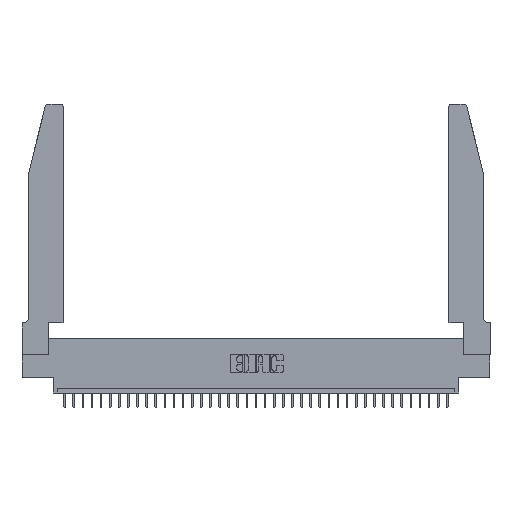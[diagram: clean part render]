
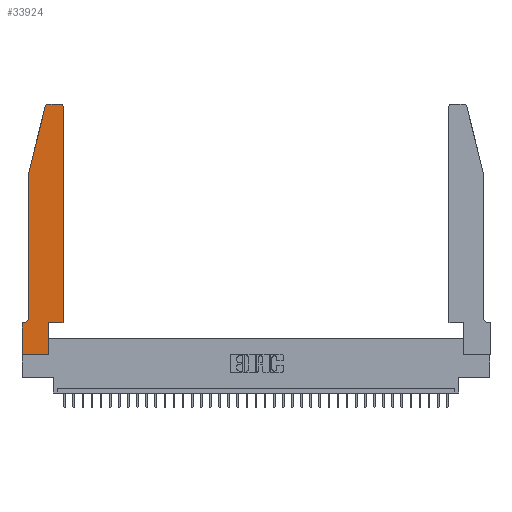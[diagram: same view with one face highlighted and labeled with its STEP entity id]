
A CAD part, top view. The second image highlights one B-rep face of the part: STEP entity #33924.
In plain terms, the highlighted planar face has unit normal (0, 0, 1).
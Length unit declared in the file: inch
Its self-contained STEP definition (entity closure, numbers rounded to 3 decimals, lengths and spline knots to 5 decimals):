
#846 = VECTOR ( 'NONE', #14399, 39.37008 ) ;
#1348 = LINE ( 'NONE', #17926, #846 ) ;
#2010 = EDGE_CURVE ( 'NONE', #20966, #9836, #18741, .T. ) ;
#2054 = CARTESIAN_POINT ( 'NONE',  ( 0.4205, 2.75, 0.37 ) ) ;
#2552 = LINE ( 'NONE', #18133, #14204 ) ;
#2618 = CARTESIAN_POINT ( 'NONE',  ( 0.0055, 0.35, 0.37 ) ) ;
#2732 = AXIS2_PLACEMENT_3D ( 'NONE', #2826, #20329, #20874 ) ;
#2826 = CARTESIAN_POINT ( 'NONE',  ( 0.4205, 2.72, 0.37 ) ) ;
#3093 = VECTOR ( 'NONE', #26132, 39.37008 ) ;
#3530 = CARTESIAN_POINT ( 'NONE',  ( 0.284, 2.75, 0.37 ) ) ;
#3638 = ORIENTED_EDGE ( 'NONE', *, *, #16015, .T. ) ;
#3653 = EDGE_CURVE ( 'NONE', #21396, #20966, #22659, .T. ) ;
#4939 = CARTESIAN_POINT ( 'NONE',  ( 0.2865, 0.35, 0.37 ) ) ;
#5002 = CIRCLE ( 'NONE', #24371, 0.03 ) ;
#5201 = ORIENTED_EDGE ( 'NONE', *, *, #29090, .T. ) ;
#6491 = LINE ( 'NONE', #16230, #36159 ) ;
#6563 = DIRECTION ( 'NONE',  ( 1., 0., 0. ) ) ;
#7030 = ORIENTED_EDGE ( 'NONE', *, *, #3653, .T. ) ;
#7491 = CARTESIAN_POINT ( 'NONE',  ( 0.25487, 2.72718, 0.37 ) ) ;
#7581 = EDGE_CURVE ( 'NONE', #14139, #18586, #10402, .T. ) ;
#7671 = VERTEX_POINT ( 'NONE', #10787 ) ;
#7734 = DIRECTION ( 'NONE',  ( 0., 1., 0. ) ) ;
#7738 = VECTOR ( 'NONE', #16692, 39.37008 ) ;
#8858 = ORIENTED_EDGE ( 'NONE', *, *, #12241, .T. ) ;
#9411 = EDGE_CURVE ( 'NONE', #30691, #10768, #2552, .T. ) ;
#9836 = VERTEX_POINT ( 'NONE', #35978 ) ;
#10402 = LINE ( 'NONE', #25443, #3093 ) ;
#10768 = VERTEX_POINT ( 'NONE', #25548 ) ;
#10787 = CARTESIAN_POINT ( 'NONE',  ( 0.0755, 2., 0.37 ) ) ;
#10963 = DIRECTION ( 'NONE',  ( 0., -1., 0. ) ) ;
#12241 = EDGE_CURVE ( 'NONE', #14148, #30691, #15282, .T. ) ;
#13136 = LINE ( 'NONE', #33552, #36939 ) ;
#13427 = EDGE_CURVE ( 'NONE', #31234, #14148, #1348, .T. ) ;
#14139 = VERTEX_POINT ( 'NONE', #2054 ) ;
#14148 = VERTEX_POINT ( 'NONE', #20504 ) ;
#14204 = VECTOR ( 'NONE', #6563, 39.37008 ) ;
#14399 = DIRECTION ( 'NONE',  ( 1., 0., 0. ) ) ;
#14471 = EDGE_CURVE ( 'NONE', #7671, #21396, #21504, .T. ) ;
#14508 = VERTEX_POINT ( 'NONE', #20963 ) ;
#14814 = CARTESIAN_POINT ( 'NONE',  ( 0.0055, 0.42, 0.37 ) ) ;
#14862 = DIRECTION ( 'NONE',  ( 1., 0., 0. ) ) ;
#15282 = LINE ( 'NONE', #33873, #7738 ) ;
#15508 = VERTEX_POINT ( 'NONE', #7491 ) ;
#15615 = VECTOR ( 'NONE', #35122, 39.37008 ) ;
#16015 = EDGE_CURVE ( 'NONE', #9836, #31234, #6491, .T. ) ;
#16161 = EDGE_LOOP ( 'NONE', ( #34150, #5201, #18253, #31601, #7030, #31455, #3638, #17999, #8858, #21811, #25681, #17723 ) ) ;
#16230 = CARTESIAN_POINT ( 'NONE',  ( 0., 0., 0.37 ) ) ;
#16692 = DIRECTION ( 'NONE',  ( 0., 1., 0. ) ) ;
#16913 = VECTOR ( 'NONE', #36275, 39.37008 ) ;
#17723 = ORIENTED_EDGE ( 'NONE', *, *, #20002, .T. ) ;
#17926 = CARTESIAN_POINT ( 'NONE',  ( 0., 0., 0.37 ) ) ;
#17999 = ORIENTED_EDGE ( 'NONE', *, *, #13427, .T. ) ;
#18133 = CARTESIAN_POINT ( 'NONE',  ( 0.4505, 0.35, 0.37 ) ) ;
#18253 = ORIENTED_EDGE ( 'NONE', *, *, #36047, .T. ) ;
#18329 = CARTESIAN_POINT ( 'NONE',  ( 0.0755, 2., 0.37 ) ) ;
#18429 = CARTESIAN_POINT ( 'NONE',  ( 0.0755, 0.42, 0.37 ) ) ;
#18456 = DIRECTION ( 'NONE',  ( -0.239, -0.971, 0. ) ) ;
#18586 = VERTEX_POINT ( 'NONE', #3530 ) ;
#18741 = LINE ( 'NONE', #33373, #16913 ) ;
#19409 = AXIS2_PLACEMENT_3D ( 'NONE', #34459, #31482, #19848 ) ;
#19724 = CIRCLE ( 'NONE', #2732, 0.03 ) ;
#19848 = DIRECTION ( 'NONE',  ( 1., 0., 0. ) ) ;
#20002 = EDGE_CURVE ( 'NONE', #14508, #14139, #19724, .T. ) ;
#20211 = AXIS2_PLACEMENT_3D ( 'NONE', #14814, #29004, #35161 ) ;
#20329 = DIRECTION ( 'NONE',  ( 0., 0., 1. ) ) ;
#20504 = CARTESIAN_POINT ( 'NONE',  ( 0.2865, 0., 0.37 ) ) ;
#20874 = DIRECTION ( 'NONE',  ( 1., 0., 0. ) ) ;
#20963 = CARTESIAN_POINT ( 'NONE',  ( 0.4505, 2.72, 0.37 ) ) ;
#20966 = VERTEX_POINT ( 'NONE', #2618 ) ;
#21396 = VERTEX_POINT ( 'NONE', #18429 ) ;
#21504 = LINE ( 'NONE', #23589, #15615 ) ;
#21811 = ORIENTED_EDGE ( 'NONE', *, *, #9411, .T. ) ;
#22659 = CIRCLE ( 'NONE', #20211, 0.07 ) ;
#23199 = FACE_OUTER_BOUND ( 'NONE', #16161, .T. ) ;
#23278 = CARTESIAN_POINT ( 'NONE',  ( 0., 0., 0.37 ) ) ;
#23589 = CARTESIAN_POINT ( 'NONE',  ( 0.0755, 2., 0.37 ) ) ;
#23959 = VECTOR ( 'NONE', #18456, 39.37008 ) ;
#24371 = AXIS2_PLACEMENT_3D ( 'NONE', #35469, #35205, #14862 ) ;
#25443 = CARTESIAN_POINT ( 'NONE',  ( 0.2605, 2.75, 0.37 ) ) ;
#25548 = CARTESIAN_POINT ( 'NONE',  ( 0.4505, 0.35, 0.37 ) ) ;
#25681 = ORIENTED_EDGE ( 'NONE', *, *, #28455, .T. ) ;
#26132 = DIRECTION ( 'NONE',  ( -1., 0., 0. ) ) ;
#28455 = EDGE_CURVE ( 'NONE', #10768, #14508, #13136, .T. ) ;
#29004 = DIRECTION ( 'NONE',  ( 0., 0., -1. ) ) ;
#29090 = EDGE_CURVE ( 'NONE', #18586, #15508, #5002, .T. ) ;
#30691 = VERTEX_POINT ( 'NONE', #4939 ) ;
#31234 = VERTEX_POINT ( 'NONE', #23278 ) ;
#31455 = ORIENTED_EDGE ( 'NONE', *, *, #2010, .T. ) ;
#31482 = DIRECTION ( 'NONE',  ( 0., 0., 1. ) ) ;
#31601 = ORIENTED_EDGE ( 'NONE', *, *, #14471, .T. ) ;
#33373 = CARTESIAN_POINT ( 'NONE',  ( 0.0755, 0.35, 0.37 ) ) ;
#33552 = CARTESIAN_POINT ( 'NONE',  ( 0.4505, 0.35, 0.37 ) ) ;
#33873 = CARTESIAN_POINT ( 'NONE',  ( 0.2865, 0.35, 0.37 ) ) ;
#33924 = ADVANCED_FACE ( 'NONE', ( #23199 ), #37167, .T. ) ;
#34150 = ORIENTED_EDGE ( 'NONE', *, *, #7581, .T. ) ;
#34459 = CARTESIAN_POINT ( 'NONE',  ( 0., 0.35, 0.37 ) ) ;
#35122 = DIRECTION ( 'NONE',  ( 0., -1., 0. ) ) ;
#35145 = LINE ( 'NONE', #18329, #23959 ) ;
#35161 = DIRECTION ( 'NONE',  ( -1., 0., 0. ) ) ;
#35205 = DIRECTION ( 'NONE',  ( 0., 0., 1. ) ) ;
#35469 = CARTESIAN_POINT ( 'NONE',  ( 0.284, 2.72, 0.37 ) ) ;
#35978 = CARTESIAN_POINT ( 'NONE',  ( 0., 0.35, 0.37 ) ) ;
#36047 = EDGE_CURVE ( 'NONE', #15508, #7671, #35145, .T. ) ;
#36159 = VECTOR ( 'NONE', #10963, 39.37008 ) ;
#36275 = DIRECTION ( 'NONE',  ( -1., 0., 0. ) ) ;
#36939 = VECTOR ( 'NONE', #7734, 39.37008 ) ;
#37167 = PLANE ( 'NONE',  #19409 ) ;
